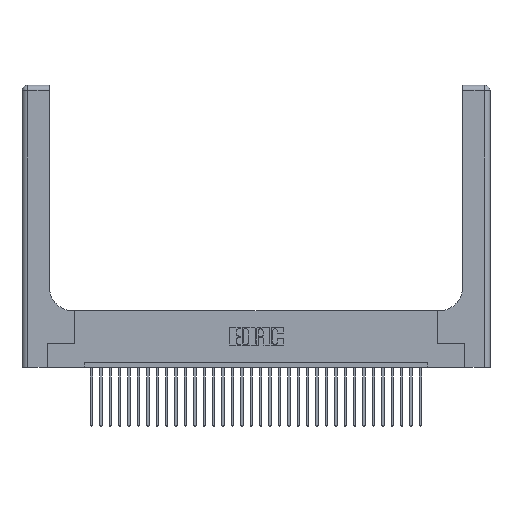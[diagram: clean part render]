
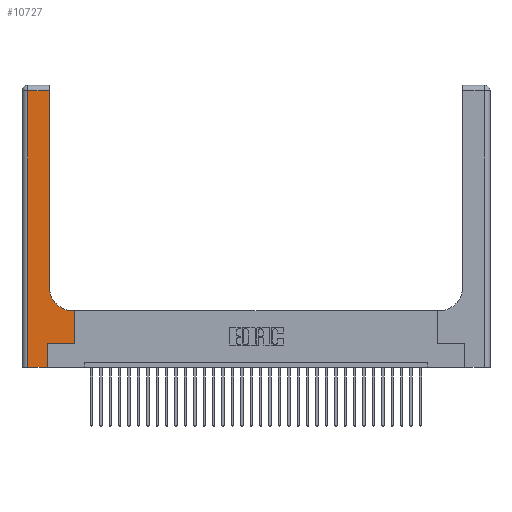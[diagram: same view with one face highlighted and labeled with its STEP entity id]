
A CAD part, top view. The second image highlights one B-rep face of the part: STEP entity #10727.
In plain terms, the highlighted planar face has unit normal (0, 0, 1).
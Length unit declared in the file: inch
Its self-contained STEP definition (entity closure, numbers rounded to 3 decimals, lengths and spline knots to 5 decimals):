
#187 = CARTESIAN_POINT ( 'NONE',  ( 0.2915, 2.94, 0.37 ) ) ;
#1078 = DIRECTION ( 'NONE',  ( 0., 1., 0. ) ) ;
#1226 = CARTESIAN_POINT ( 'NONE',  ( 0.06, 2.94, 0.37 ) ) ;
#1384 = VECTOR ( 'NONE', #3263, 39.37008 ) ;
#1594 = VERTEX_POINT ( 'NONE', #1226 ) ;
#1746 = CARTESIAN_POINT ( 'NONE',  ( 0.5585, 0.6, 0.37 ) ) ;
#3050 = EDGE_CURVE ( 'NONE', #12920, #16860, #13571, .T. ) ;
#3126 = VERTEX_POINT ( 'NONE', #12982 ) ;
#3263 = DIRECTION ( 'NONE',  ( -1., 0., 0. ) ) ;
#3410 = CARTESIAN_POINT ( 'NONE',  ( 0.5585, 0.25, 0.37 ) ) ;
#3591 = DIRECTION ( 'NONE',  ( 0., -1., 0. ) ) ;
#3938 = EDGE_CURVE ( 'NONE', #25630, #13942, #10526, .T. ) ;
#4113 = DIRECTION ( 'NONE',  ( -1., 0., 0. ) ) ;
#4886 = DIRECTION ( 'NONE',  ( 1., 0., 0. ) ) ;
#4999 = LINE ( 'NONE', #27399, #12261 ) ;
#5084 = EDGE_CURVE ( 'NONE', #16860, #1594, #8859, .T. ) ;
#5243 = CARTESIAN_POINT ( 'NONE',  ( 0.5585, 0.25, 0.37 ) ) ;
#5942 = CARTESIAN_POINT ( 'NONE',  ( 0.269, 0., 0.37 ) ) ;
#6542 = EDGE_CURVE ( 'NONE', #13942, #13169, #12020, .T. ) ;
#6590 = CARTESIAN_POINT ( 'NONE',  ( 0., 3., 0.37 ) ) ;
#6831 = DIRECTION ( 'NONE',  ( 0., 0., -1. ) ) ;
#7667 = EDGE_CURVE ( 'NONE', #8406, #12920, #20652, .T. ) ;
#7951 = ORIENTED_EDGE ( 'NONE', *, *, #3050, .T. ) ;
#8372 = EDGE_LOOP ( 'NONE', ( #7951, #13683, #27053, #12547, #16758, #25880, #28812, #21810, #33005 ) ) ;
#8406 = VERTEX_POINT ( 'NONE', #16365 ) ;
#8531 = CARTESIAN_POINT ( 'NONE',  ( 0.2915, 0.6, 0.37 ) ) ;
#8600 = DIRECTION ( 'NONE',  ( 0., 1., 0. ) ) ;
#8859 = LINE ( 'NONE', #13843, #23623 ) ;
#10526 = LINE ( 'NONE', #5942, #27332 ) ;
#10646 = CARTESIAN_POINT ( 'NONE',  ( 0.06, 3., 0.37 ) ) ;
#10700 = EDGE_CURVE ( 'NONE', #3126, #25630, #4999, .T. ) ;
#10727 = ADVANCED_FACE ( 'NONE', ( #28566 ), #32014, .F. ) ;
#11195 = AXIS2_PLACEMENT_3D ( 'NONE', #6590, #6831, #4113 ) ;
#12020 = LINE ( 'NONE', #17211, #23169 ) ;
#12261 = VECTOR ( 'NONE', #15246, 39.37008 ) ;
#12547 = ORIENTED_EDGE ( 'NONE', *, *, #10700, .T. ) ;
#12920 = VERTEX_POINT ( 'NONE', #27371 ) ;
#12982 = CARTESIAN_POINT ( 'NONE',  ( 0.06, 0., 0.37 ) ) ;
#13169 = VERTEX_POINT ( 'NONE', #3410 ) ;
#13229 = LINE ( 'NONE', #10646, #21620 ) ;
#13532 = DIRECTION ( 'NONE',  ( 0., 1., 0. ) ) ;
#13571 = LINE ( 'NONE', #15650, #19572 ) ;
#13683 = ORIENTED_EDGE ( 'NONE', *, *, #5084, .T. ) ;
#13843 = CARTESIAN_POINT ( 'NONE',  ( 0., 2.94, 0.37 ) ) ;
#13942 = VERTEX_POINT ( 'NONE', #27196 ) ;
#14973 = DIRECTION ( 'NONE',  ( -1., 0., 0. ) ) ;
#15246 = DIRECTION ( 'NONE',  ( 1., 0., 0. ) ) ;
#15650 = CARTESIAN_POINT ( 'NONE',  ( 0.2915, 3., 0.37 ) ) ;
#16365 = CARTESIAN_POINT ( 'NONE',  ( 0.5415, 0.6, 0.37 ) ) ;
#16758 = ORIENTED_EDGE ( 'NONE', *, *, #3938, .T. ) ;
#16848 = EDGE_CURVE ( 'NONE', #13169, #25193, #20252, .T. ) ;
#16860 = VERTEX_POINT ( 'NONE', #187 ) ;
#17015 = LINE ( 'NONE', #8531, #1384 ) ;
#17211 = CARTESIAN_POINT ( 'NONE',  ( 0.269, 0.25, 0.37 ) ) ;
#17496 = VECTOR ( 'NONE', #13532, 39.37008 ) ;
#17546 = DIRECTION ( 'NONE',  ( 1., 0., 0. ) ) ;
#19572 = VECTOR ( 'NONE', #1078, 39.37008 ) ;
#20252 = LINE ( 'NONE', #5243, #17496 ) ;
#20430 = DIRECTION ( 'NONE',  ( 0., 0., -1. ) ) ;
#20652 = CIRCLE ( 'NONE', #32299, 0.25 ) ;
#20705 = EDGE_CURVE ( 'NONE', #1594, #3126, #13229, .T. ) ;
#21620 = VECTOR ( 'NONE', #3591, 39.37008 ) ;
#21810 = ORIENTED_EDGE ( 'NONE', *, *, #30068, .T. ) ;
#23169 = VECTOR ( 'NONE', #17546, 39.37008 ) ;
#23623 = VECTOR ( 'NONE', #14973, 39.37008 ) ;
#25193 = VERTEX_POINT ( 'NONE', #1746 ) ;
#25250 = CARTESIAN_POINT ( 'NONE',  ( 0.5415, 0.85, 0.37 ) ) ;
#25630 = VERTEX_POINT ( 'NONE', #31378 ) ;
#25880 = ORIENTED_EDGE ( 'NONE', *, *, #6542, .T. ) ;
#27053 = ORIENTED_EDGE ( 'NONE', *, *, #20705, .T. ) ;
#27196 = CARTESIAN_POINT ( 'NONE',  ( 0.269, 0.25, 0.37 ) ) ;
#27332 = VECTOR ( 'NONE', #8600, 39.37008 ) ;
#27371 = CARTESIAN_POINT ( 'NONE',  ( 0.2915, 0.85, 0.37 ) ) ;
#27399 = CARTESIAN_POINT ( 'NONE',  ( 0., 0., 0.37 ) ) ;
#28566 = FACE_OUTER_BOUND ( 'NONE', #8372, .T. ) ;
#28812 = ORIENTED_EDGE ( 'NONE', *, *, #16848, .T. ) ;
#30068 = EDGE_CURVE ( 'NONE', #25193, #8406, #17015, .T. ) ;
#31378 = CARTESIAN_POINT ( 'NONE',  ( 0.269, 0., 0.37 ) ) ;
#32014 = PLANE ( 'NONE',  #11195 ) ;
#32299 = AXIS2_PLACEMENT_3D ( 'NONE', #25250, #20430, #4886 ) ;
#33005 = ORIENTED_EDGE ( 'NONE', *, *, #7667, .T. ) ;
